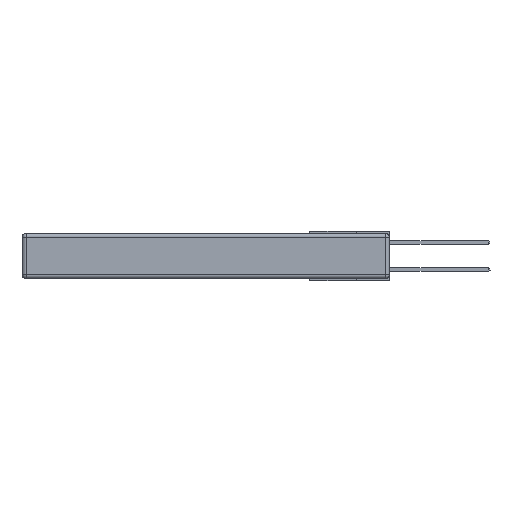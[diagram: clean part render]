
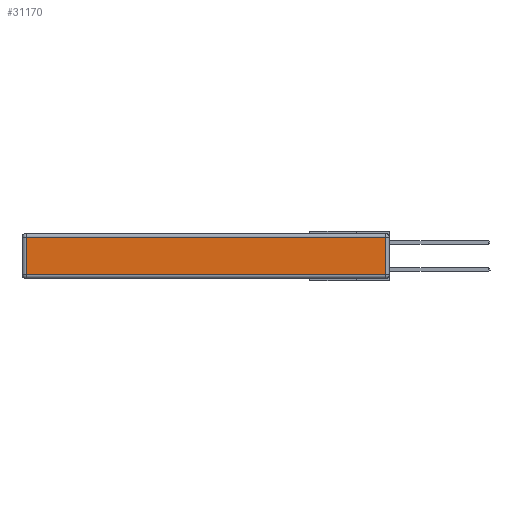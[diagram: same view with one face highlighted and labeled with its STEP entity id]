
A CAD part, left-side view. The second image highlights one B-rep face of the part: STEP entity #31170.
In plain terms, the highlighted planar face has unit normal (-1, 0, 0).
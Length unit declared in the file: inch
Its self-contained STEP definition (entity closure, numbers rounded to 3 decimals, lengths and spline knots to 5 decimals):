
#256 = ORIENTED_EDGE ( 'NONE', *, *, #14648, .T. ) ;
#1450 = CARTESIAN_POINT ( 'NONE',  ( 0., 2.72, -0.313 ) ) ;
#3605 = ORIENTED_EDGE ( 'NONE', *, *, #22065, .T. ) ;
#3758 = ORIENTED_EDGE ( 'NONE', *, *, #24010, .T. ) ;
#4060 = CARTESIAN_POINT ( 'NONE',  ( 0., 0., -0.313 ) ) ;
#4609 = EDGE_CURVE ( 'NONE', #21799, #8285, #26009, .T. ) ;
#4882 = CARTESIAN_POINT ( 'NONE',  ( 0., 0.03, -0.313 ) ) ;
#8285 = VERTEX_POINT ( 'NONE', #4882 ) ;
#8827 = DIRECTION ( 'NONE',  ( 0., 0., -1. ) ) ;
#9028 = DIRECTION ( 'NONE',  ( 0., 0., 1. ) ) ;
#9102 = VECTOR ( 'NONE', #28750, 39.37008 ) ;
#10015 = LINE ( 'NONE', #22075, #29443 ) ;
#10539 = VECTOR ( 'NONE', #32194, 39.37008 ) ;
#10997 = CARTESIAN_POINT ( 'NONE',  ( 0., 2.75, -0.03 ) ) ;
#11498 = LINE ( 'NONE', #14225, #17413 ) ;
#12282 = VERTEX_POINT ( 'NONE', #17141 ) ;
#14225 = CARTESIAN_POINT ( 'NONE',  ( 0., 2.72, -0.343 ) ) ;
#14648 = EDGE_CURVE ( 'NONE', #22595, #12282, #23353, .T. ) ;
#17141 = CARTESIAN_POINT ( 'NONE',  ( 0., 2.72, -0.03 ) ) ;
#17413 = VECTOR ( 'NONE', #8827, 39.37008 ) ;
#18729 = FACE_OUTER_BOUND ( 'NONE', #27876, .T. ) ;
#19292 = CARTESIAN_POINT ( 'NONE',  ( 0., 0.03, -0.03 ) ) ;
#20961 = DIRECTION ( 'NONE',  ( -1., 0., 0. ) ) ;
#21799 = VERTEX_POINT ( 'NONE', #1450 ) ;
#22065 = EDGE_CURVE ( 'NONE', #8285, #22595, #10015, .T. ) ;
#22075 = CARTESIAN_POINT ( 'NONE',  ( 0., 0.03, -0.343 ) ) ;
#22595 = VERTEX_POINT ( 'NONE', #19292 ) ;
#23353 = LINE ( 'NONE', #10997, #9102 ) ;
#24010 = EDGE_CURVE ( 'NONE', #12282, #21799, #11498, .T. ) ;
#24192 = CARTESIAN_POINT ( 'NONE',  ( 0., 0., -0.343 ) ) ;
#26009 = LINE ( 'NONE', #4060, #10539 ) ;
#26631 = ORIENTED_EDGE ( 'NONE', *, *, #4609, .T. ) ;
#26905 = AXIS2_PLACEMENT_3D ( 'NONE', #24192, #20961, #9028 ) ;
#27134 = DIRECTION ( 'NONE',  ( 0., 0., 1. ) ) ;
#27876 = EDGE_LOOP ( 'NONE', ( #26631, #3605, #256, #3758 ) ) ;
#28750 = DIRECTION ( 'NONE',  ( 0., 1., 0. ) ) ;
#29443 = VECTOR ( 'NONE', #27134, 39.37008 ) ;
#31170 = ADVANCED_FACE ( 'NONE', ( #18729 ), #31860, .T. ) ;
#31860 = PLANE ( 'NONE',  #26905 ) ;
#32194 = DIRECTION ( 'NONE',  ( 0., -1., 0. ) ) ;
